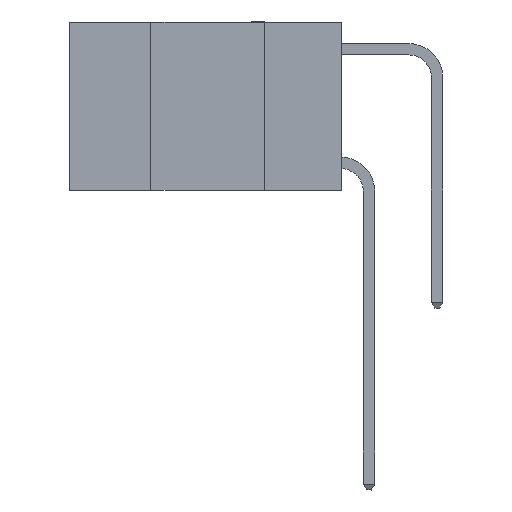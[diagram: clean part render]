
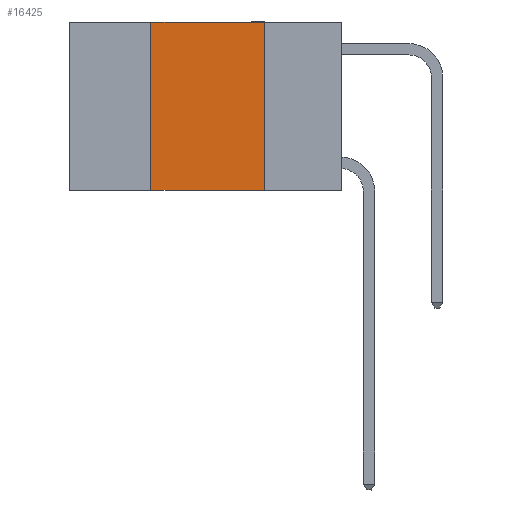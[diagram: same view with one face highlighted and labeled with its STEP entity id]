
A CAD part, left-side view. The second image highlights one B-rep face of the part: STEP entity #16425.
In plain terms, the highlighted planar face has unit normal (-1, 0, 0).
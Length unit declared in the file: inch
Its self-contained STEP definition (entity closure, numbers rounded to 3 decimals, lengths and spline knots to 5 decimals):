
#582 = CARTESIAN_POINT ( 'NONE',  ( 0., 0.6, -0.37 ) ) ;
#1539 = EDGE_CURVE ( 'NONE', #13002, #21771, #17859, .T. ) ;
#2755 = CARTESIAN_POINT ( 'NONE',  ( 0., 0.6, 0. ) ) ;
#3668 = VERTEX_POINT ( 'NONE', #14451 ) ;
#4331 = DIRECTION ( 'NONE',  ( 0., 0., 1. ) ) ;
#4552 = DIRECTION ( 'NONE',  ( 1., 0., 0. ) ) ;
#4625 = CARTESIAN_POINT ( 'NONE',  ( 0., 0.17, -0.37 ) ) ;
#4995 = CARTESIAN_POINT ( 'NONE',  ( 0., 0.17, 0. ) ) ;
#5145 = EDGE_CURVE ( 'NONE', #13002, #23063, #6008, .T. ) ;
#5704 = LINE ( 'NONE', #6602, #19915 ) ;
#6008 = LINE ( 'NONE', #13251, #14947 ) ;
#6213 = ORIENTED_EDGE ( 'NONE', *, *, #5145, .F. ) ;
#6602 = CARTESIAN_POINT ( 'NONE',  ( 0., 0.6, 0. ) ) ;
#7537 = EDGE_CURVE ( 'NONE', #3668, #21771, #22454, .T. ) ;
#9859 = PLANE ( 'NONE',  #21103 ) ;
#12202 = DIRECTION ( 'NONE',  ( 0., 0., -1. ) ) ;
#12961 = FACE_OUTER_BOUND ( 'NONE', #14053, .T. ) ;
#13002 = VERTEX_POINT ( 'NONE', #18107 ) ;
#13004 = VECTOR ( 'NONE', #12202, 39.37008 ) ;
#13140 = VECTOR ( 'NONE', #18161, 39.37008 ) ;
#13251 = CARTESIAN_POINT ( 'NONE',  ( 0., 0.42, 0. ) ) ;
#14053 = EDGE_LOOP ( 'NONE', ( #22708, #16828, #6213, #15437 ) ) ;
#14451 = CARTESIAN_POINT ( 'NONE',  ( 0., 0.17, 0. ) ) ;
#14947 = VECTOR ( 'NONE', #4331, 39.37008 ) ;
#15437 = ORIENTED_EDGE ( 'NONE', *, *, #1539, .T. ) ;
#16425 = ADVANCED_FACE ( 'NONE', ( #12961 ), #9859, .F. ) ;
#16828 = ORIENTED_EDGE ( 'NONE', *, *, #21276, .F. ) ;
#17037 = DIRECTION ( 'NONE',  ( 0., 0., -1. ) ) ;
#17859 = LINE ( 'NONE', #582, #13140 ) ;
#18107 = CARTESIAN_POINT ( 'NONE',  ( 0., 0.42, -0.37 ) ) ;
#18161 = DIRECTION ( 'NONE',  ( 0., -1., 0. ) ) ;
#19057 = DIRECTION ( 'NONE',  ( 0., -1., 0. ) ) ;
#19915 = VECTOR ( 'NONE', #19057, 39.37008 ) ;
#21103 = AXIS2_PLACEMENT_3D ( 'NONE', #2755, #4552, #17037 ) ;
#21276 = EDGE_CURVE ( 'NONE', #23063, #3668, #5704, .T. ) ;
#21771 = VERTEX_POINT ( 'NONE', #4625 ) ;
#22197 = CARTESIAN_POINT ( 'NONE',  ( 0., 0.42, 0. ) ) ;
#22454 = LINE ( 'NONE', #4995, #13004 ) ;
#22708 = ORIENTED_EDGE ( 'NONE', *, *, #7537, .F. ) ;
#23063 = VERTEX_POINT ( 'NONE', #22197 ) ;
